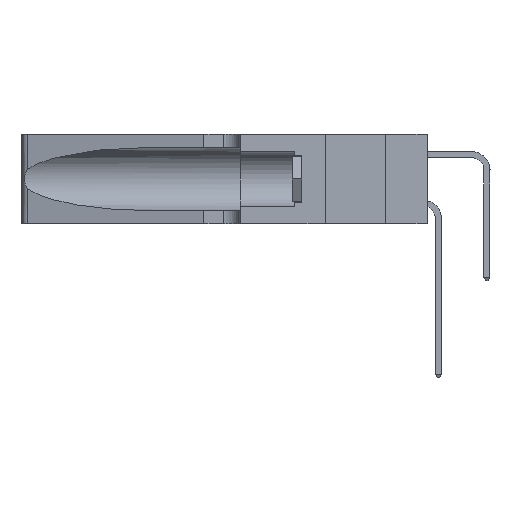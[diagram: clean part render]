
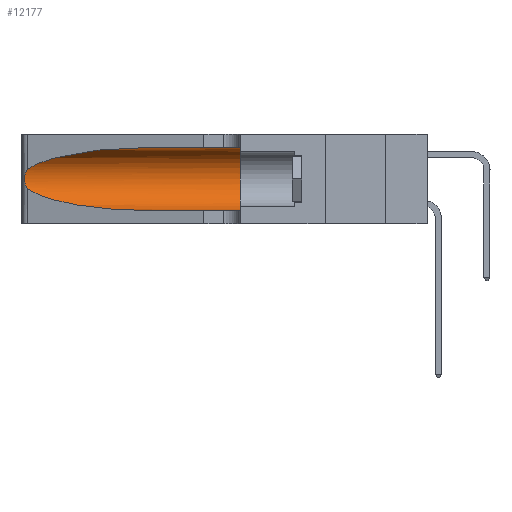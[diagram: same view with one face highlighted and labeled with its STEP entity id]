
A CAD part, left-side view. The second image highlights one B-rep face of the part: STEP entity #12177.
In plain terms, the highlighted cylindrical face has radius 3.308 mm (diameter 6.617 mm), a partial arc.
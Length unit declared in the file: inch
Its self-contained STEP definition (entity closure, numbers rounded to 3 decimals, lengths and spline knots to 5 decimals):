
#535 = CARTESIAN_POINT ( 'NONE',  ( 0.25487, 1.22718, 0.22369 ) ) ;
#1366 = CARTESIAN_POINT ( 'NONE',  ( 0.2373, 1.15595, 0.08982 ) ) ;
#1645 = CARTESIAN_POINT ( 'NONE',  ( 0.25639, 1.23186, 0.15144 ) ) ;
#2103 = CARTESIAN_POINT ( 'NONE',  ( 0.25856, 1.23593, 0.16098 ) ) ;
#2791 = CARTESIAN_POINT ( 'NONE',  ( 0.18966, 0.96281, 0.31525 ) ) ;
#3769 = VERTEX_POINT ( 'NONE', #19467 ) ;
#4062 = CARTESIAN_POINT ( 'NONE',  ( 0.25555, 1.22994, 0.2215 ) ) ;
#4438 = LINE ( 'NONE', #22106, #29726 ) ;
#4868 = CARTESIAN_POINT ( 'NONE',  ( 0.1305, 0.72297, 0.05475 ) ) ;
#4925 = DIRECTION ( 'NONE',  ( 0., -1., 0. ) ) ;
#6800 = CIRCLE ( 'NONE', #33748, 0.13025 ) ;
#7325 = CARTESIAN_POINT ( 'NONE',  ( 0.25487, 1.22718, 0.22369 ) ) ;
#8498 = EDGE_CURVE ( 'NONE', #25989, #40335, #25493, .T. ) ;
#8789 = CARTESIAN_POINT ( 'NONE',  ( 0.26075, 1.23896, 0.178 ) ) ;
#9664 = VERTEX_POINT ( 'NONE', #19873 ) ;
#11092 = CARTESIAN_POINT ( 'NONE',  ( 0.25854, 1.2359, 0.20912 ) ) ;
#11562 = VERTEX_POINT ( 'NONE', #36314 ) ;
#12177 = ADVANCED_FACE ( 'NONE', ( #22488 ), #41109, .F. ) ;
#12518 = CARTESIAN_POINT ( 'NONE',  ( 0.1305, 0.72297, 0.31525 ) ) ;
#12595 = ORIENTED_EDGE ( 'NONE', *, *, #29975, .F. ) ;
#14378 = DIRECTION ( 'NONE',  ( 0., 1., 0. ) ) ;
#15843 = CARTESIAN_POINT ( 'NONE',  ( 0.25789, 1.23486, 0.15765 ) ) ;
#16619 = B_SPLINE_CURVE_WITH_KNOTS ( 'NONE', 3,
 ( #535, #4062, #35984, #22020, #11092, #26297, #40534, #8789, #29536, #2103, #15843, #1645, #26134, #19260 ),
 .UNSPECIFIED., .F., .F.,
 ( 4, 2, 2, 2, 2, 2, 4 ),
 ( 0., 0.00027, 0.00053, 0.00107, 0.0016, 0.00187, 0.00214 ),
 .UNSPECIFIED. ) ;
#17196 =( BOUNDED_CURVE ( )  B_SPLINE_CURVE ( 3, ( #36528, #2791, #28172, #25079 ),
 .UNSPECIFIED., .F., .F. ) 
 B_SPLINE_CURVE_WITH_KNOTS ( ( 4, 4 ),
 ( 1.5708, 2.84003 ),
 .UNSPECIFIED. ) 
 CURVE ( )  GEOMETRIC_REPRESENTATION_ITEM ( )  RATIONAL_B_SPLINE_CURVE ( ( 1., 0.87, 0.87, 1. ) ) 
 REPRESENTATION_ITEM ( '' )  );
#19193 =( BOUNDED_CURVE ( )  B_SPLINE_CURVE ( 3, ( #29557, #1366, #25857, #4868 ),
 .UNSPECIFIED., .F., .F. ) 
 B_SPLINE_CURVE_WITH_KNOTS ( ( 4, 4 ),
 ( 3.44316, 4.71239 ),
 .UNSPECIFIED. ) 
 CURVE ( )  GEOMETRIC_REPRESENTATION_ITEM ( )  RATIONAL_B_SPLINE_CURVE ( ( 1., 0.87, 0.87, 1. ) ) 
 REPRESENTATION_ITEM ( '' )  );
#19260 = CARTESIAN_POINT ( 'NONE',  ( 0.25487, 1.22718, 0.14631 ) ) ;
#19467 = CARTESIAN_POINT ( 'NONE',  ( 0.1305, 0.35, 0.05475 ) ) ;
#19873 = CARTESIAN_POINT ( 'NONE',  ( 0.1305, 0.72297, 0.05475 ) ) ;
#20047 = CARTESIAN_POINT ( 'NONE',  ( 0.1305, 0.35, 0.31525 ) ) ;
#20450 = DIRECTION ( 'NONE',  ( 0., -1., 0. ) ) ;
#22020 = CARTESIAN_POINT ( 'NONE',  ( 0.25787, 1.23484, 0.2124 ) ) ;
#22106 = CARTESIAN_POINT ( 'NONE',  ( 0.1305, 1.61858, 0.05475 ) ) ;
#22488 = FACE_OUTER_BOUND ( 'NONE', #29635, .T. ) ;
#23529 = DIRECTION ( 'NONE',  ( 0., 0., -1. ) ) ;
#24423 = AXIS2_PLACEMENT_3D ( 'NONE', #34431, #20450, #23529 ) ;
#25079 = CARTESIAN_POINT ( 'NONE',  ( 0.25487, 1.22718, 0.22369 ) ) ;
#25146 = EDGE_CURVE ( 'NONE', #41117, #11562, #16619, .T. ) ;
#25493 = LINE ( 'NONE', #37824, #35401 ) ;
#25857 = CARTESIAN_POINT ( 'NONE',  ( 0.18966, 0.96281, 0.05475 ) ) ;
#25989 = VERTEX_POINT ( 'NONE', #12518 ) ;
#26134 = CARTESIAN_POINT ( 'NONE',  ( 0.25555, 1.22993, 0.14849 ) ) ;
#26297 = CARTESIAN_POINT ( 'NONE',  ( 0.26018, 1.23835, 0.19895 ) ) ;
#28090 = DIRECTION ( 'NONE',  ( 0., 0., 1. ) ) ;
#28172 = CARTESIAN_POINT ( 'NONE',  ( 0.2373, 1.15595, 0.28018 ) ) ;
#28433 = ORIENTED_EDGE ( 'NONE', *, *, #43319, .T. ) ;
#29536 = CARTESIAN_POINT ( 'NONE',  ( 0.26017, 1.23833, 0.17102 ) ) ;
#29557 = CARTESIAN_POINT ( 'NONE',  ( 0.25487, 1.22718, 0.14631 ) ) ;
#29635 = EDGE_LOOP ( 'NONE', ( #38771, #44347, #28433, #30062, #12595, #42040 ) ) ;
#29726 = VECTOR ( 'NONE', #4925, 39.37008 ) ;
#29975 = EDGE_CURVE ( 'NONE', #40335, #3769, #6800, .T. ) ;
#30062 = ORIENTED_EDGE ( 'NONE', *, *, #31906, .T. ) ;
#30111 = EDGE_CURVE ( 'NONE', #25989, #41117, #17196, .T. ) ;
#31906 = EDGE_CURVE ( 'NONE', #9664, #3769, #4438, .T. ) ;
#33748 = AXIS2_PLACEMENT_3D ( 'NONE', #35453, #14378, #28090 ) ;
#34431 = CARTESIAN_POINT ( 'NONE',  ( 0.1305, 1.61858, 0.185 ) ) ;
#35401 = VECTOR ( 'NONE', #41146, 39.37008 ) ;
#35453 = CARTESIAN_POINT ( 'NONE',  ( 0.1305, 0.35, 0.185 ) ) ;
#35984 = CARTESIAN_POINT ( 'NONE',  ( 0.25639, 1.23184, 0.21858 ) ) ;
#36314 = CARTESIAN_POINT ( 'NONE',  ( 0.25487, 1.22718, 0.14631 ) ) ;
#36528 = CARTESIAN_POINT ( 'NONE',  ( 0.1305, 0.72297, 0.31525 ) ) ;
#37824 = CARTESIAN_POINT ( 'NONE',  ( 0.1305, 1.61858, 0.31525 ) ) ;
#38771 = ORIENTED_EDGE ( 'NONE', *, *, #30111, .T. ) ;
#40335 = VERTEX_POINT ( 'NONE', #20047 ) ;
#40534 = CARTESIAN_POINT ( 'NONE',  ( 0.26075, 1.23896, 0.19203 ) ) ;
#41109 = CYLINDRICAL_SURFACE ( 'NONE', #24423, 0.13025 ) ;
#41117 = VERTEX_POINT ( 'NONE', #7325 ) ;
#41146 = DIRECTION ( 'NONE',  ( 0., -1., 0. ) ) ;
#42040 = ORIENTED_EDGE ( 'NONE', *, *, #8498, .F. ) ;
#43319 = EDGE_CURVE ( 'NONE', #11562, #9664, #19193, .T. ) ;
#44347 = ORIENTED_EDGE ( 'NONE', *, *, #25146, .T. ) ;
